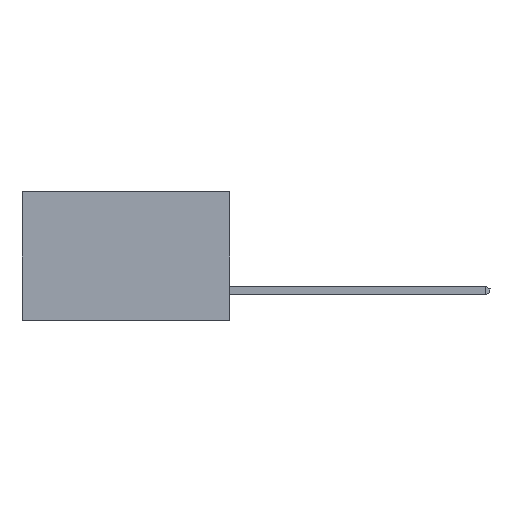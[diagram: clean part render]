
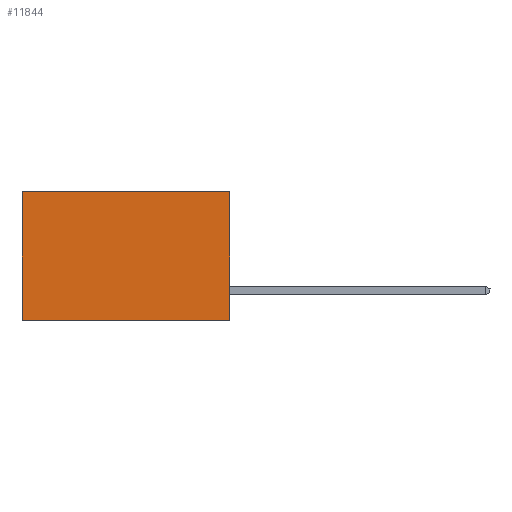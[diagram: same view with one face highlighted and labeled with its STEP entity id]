
A CAD part, left-side view. The second image highlights one B-rep face of the part: STEP entity #11844.
In plain terms, the highlighted planar face has unit normal (-1, 0, 0).
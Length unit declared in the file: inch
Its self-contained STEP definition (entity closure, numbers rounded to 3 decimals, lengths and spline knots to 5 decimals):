
#278 = CARTESIAN_POINT ( 'NONE',  ( 0.2615, 0., 0. ) ) ;
#915 = VERTEX_POINT ( 'NONE', #7059 ) ;
#1204 = VECTOR ( 'NONE', #8525, 39.37008 ) ;
#2095 = EDGE_CURVE ( 'NONE', #6354, #16360, #3559, .T. ) ;
#2445 = EDGE_LOOP ( 'NONE', ( #4657, #9244, #15156, #3684 ) ) ;
#3559 = LINE ( 'NONE', #11999, #18493 ) ;
#3684 = ORIENTED_EDGE ( 'NONE', *, *, #11162, .T. ) ;
#3887 = VECTOR ( 'NONE', #4714, 39.37008 ) ;
#4657 = ORIENTED_EDGE ( 'NONE', *, *, #5838, .T. ) ;
#4714 = DIRECTION ( 'NONE',  ( 0., 1., 0. ) ) ;
#5838 = EDGE_CURVE ( 'NONE', #17117, #16360, #14591, .T. ) ;
#6354 = VERTEX_POINT ( 'NONE', #18182 ) ;
#6588 = FACE_OUTER_BOUND ( 'NONE', #2445, .T. ) ;
#6935 = AXIS2_PLACEMENT_3D ( 'NONE', #9459, #15225, #13713 ) ;
#7059 = CARTESIAN_POINT ( 'NONE',  ( 0.2615, 0., 0. ) ) ;
#7292 = CARTESIAN_POINT ( 'NONE',  ( 0.2615, 0., -0.37 ) ) ;
#8525 = DIRECTION ( 'NONE',  ( 0., 0., -1. ) ) ;
#8914 = LINE ( 'NONE', #278, #3887 ) ;
#9244 = ORIENTED_EDGE ( 'NONE', *, *, #2095, .F. ) ;
#9349 = DIRECTION ( 'NONE',  ( 0., 1., 0. ) ) ;
#9459 = CARTESIAN_POINT ( 'NONE',  ( 0.2615, 0., -0.37 ) ) ;
#10427 = DIRECTION ( 'NONE',  ( 0., 0., -1. ) ) ;
#11162 = EDGE_CURVE ( 'NONE', #915, #17117, #8914, .T. ) ;
#11844 = ADVANCED_FACE ( 'NONE', ( #6588 ), #16352, .F. ) ;
#11999 = CARTESIAN_POINT ( 'NONE',  ( 0.2615, 0., -0.37 ) ) ;
#12789 = EDGE_CURVE ( 'NONE', #915, #6354, #14223, .T. ) ;
#13713 = DIRECTION ( 'NONE',  ( 0., 0., -1. ) ) ;
#14223 = LINE ( 'NONE', #7292, #1204 ) ;
#14591 = LINE ( 'NONE', #17390, #15109 ) ;
#15109 = VECTOR ( 'NONE', #10427, 39.37008 ) ;
#15156 = ORIENTED_EDGE ( 'NONE', *, *, #12789, .F. ) ;
#15225 = DIRECTION ( 'NONE',  ( 1., 0., 0. ) ) ;
#15343 = CARTESIAN_POINT ( 'NONE',  ( 0.2615, 0.6, 0. ) ) ;
#16352 = PLANE ( 'NONE',  #6935 ) ;
#16360 = VERTEX_POINT ( 'NONE', #18657 ) ;
#17117 = VERTEX_POINT ( 'NONE', #15343 ) ;
#17390 = CARTESIAN_POINT ( 'NONE',  ( 0.2615, 0.6, -0.37 ) ) ;
#18182 = CARTESIAN_POINT ( 'NONE',  ( 0.2615, 0., -0.37 ) ) ;
#18493 = VECTOR ( 'NONE', #9349, 39.37008 ) ;
#18657 = CARTESIAN_POINT ( 'NONE',  ( 0.2615, 0.6, -0.37 ) ) ;
